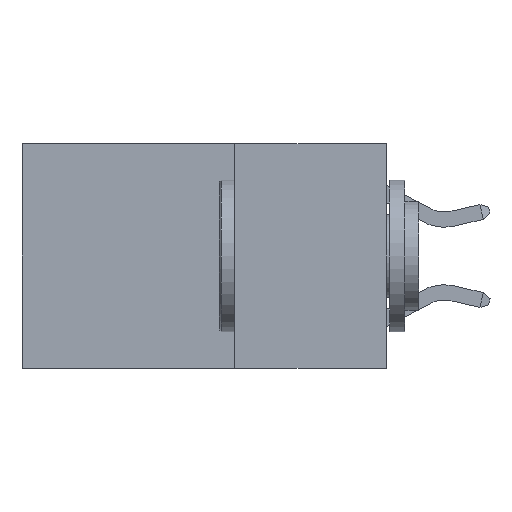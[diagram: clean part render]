
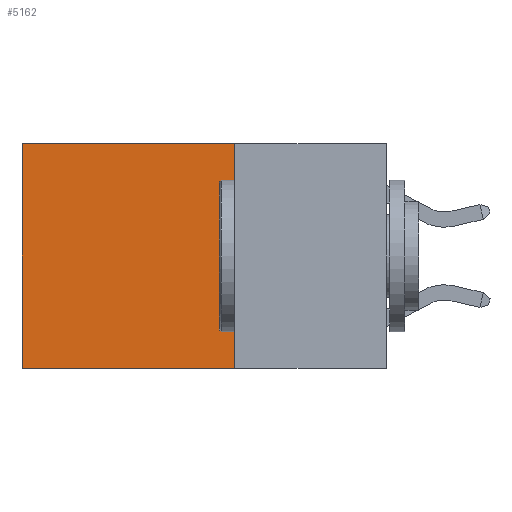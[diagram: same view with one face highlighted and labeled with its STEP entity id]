
A CAD part, left-side view. The second image highlights one B-rep face of the part: STEP entity #5162.
In plain terms, the highlighted planar face has unit normal (-1, 0, 0).
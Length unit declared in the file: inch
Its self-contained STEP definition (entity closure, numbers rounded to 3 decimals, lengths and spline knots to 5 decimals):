
#210 = EDGE_CURVE ( 'NONE', #7461, #4934, #9469, .T. ) ;
#253 = CARTESIAN_POINT ( 'NONE',  ( 0.2625, 0.25, -0.37 ) ) ;
#627 = CARTESIAN_POINT ( 'NONE',  ( 0.2625, 0.6, 0. ) ) ;
#638 = CARTESIAN_POINT ( 'NONE',  ( 0.2625, 0.6, 0. ) ) ;
#1052 = ORIENTED_EDGE ( 'NONE', *, *, #5320, .F. ) ;
#1684 = DIRECTION ( 'NONE',  ( 0., 0., -1. ) ) ;
#1700 = PLANE ( 'NONE',  #1705 ) ;
#1705 = AXIS2_PLACEMENT_3D ( 'NONE', #1714, #1871, #1684 ) ;
#1714 = CARTESIAN_POINT ( 'NONE',  ( 0.2625, 0.25, 0. ) ) ;
#1727 = VERTEX_POINT ( 'NONE', #5389 ) ;
#1871 = DIRECTION ( 'NONE',  ( 1., 0., 0. ) ) ;
#3187 = ORIENTED_EDGE ( 'NONE', *, *, #8732, .F. ) ;
#3204 = LINE ( 'NONE', #253, #3427 ) ;
#3427 = VECTOR ( 'NONE', #5504, 39.37008 ) ;
#3429 = VECTOR ( 'NONE', #3746, 39.37008 ) ;
#3746 = DIRECTION ( 'NONE',  ( 0., 1., 0. ) ) ;
#3990 = ORIENTED_EDGE ( 'NONE', *, *, #210, .T. ) ;
#4029 = CARTESIAN_POINT ( 'NONE',  ( 0.2625, 0.25, 0. ) ) ;
#4235 = DIRECTION ( 'NONE',  ( 0., 0., -1. ) ) ;
#4585 = CARTESIAN_POINT ( 'NONE',  ( 0.2625, 0.25, 0. ) ) ;
#4934 = VERTEX_POINT ( 'NONE', #8259 ) ;
#5162 = ADVANCED_FACE ( 'NONE', ( #8408 ), #1700, .F. ) ;
#5320 = EDGE_CURVE ( 'NONE', #1727, #4934, #3204, .T. ) ;
#5389 = CARTESIAN_POINT ( 'NONE',  ( 0.2625, 0.25, -0.37 ) ) ;
#5504 = DIRECTION ( 'NONE',  ( 0., 1., 0. ) ) ;
#7113 = VECTOR ( 'NONE', #7655, 39.37008 ) ;
#7322 = LINE ( 'NONE', #9468, #3429 ) ;
#7461 = VERTEX_POINT ( 'NONE', #638 ) ;
#7625 = VECTOR ( 'NONE', #4235, 39.37008 ) ;
#7630 = VERTEX_POINT ( 'NONE', #4585 ) ;
#7655 = DIRECTION ( 'NONE',  ( 0., 0., -1. ) ) ;
#8087 = EDGE_LOOP ( 'NONE', ( #3990, #1052, #3187, #8374 ) ) ;
#8259 = CARTESIAN_POINT ( 'NONE',  ( 0.2625, 0.6, -0.37 ) ) ;
#8374 = ORIENTED_EDGE ( 'NONE', *, *, #9227, .T. ) ;
#8408 = FACE_OUTER_BOUND ( 'NONE', #8087, .T. ) ;
#8732 = EDGE_CURVE ( 'NONE', #7630, #1727, #8982, .T. ) ;
#8982 = LINE ( 'NONE', #4029, #7113 ) ;
#9227 = EDGE_CURVE ( 'NONE', #7630, #7461, #7322, .T. ) ;
#9468 = CARTESIAN_POINT ( 'NONE',  ( 0.2625, 0.25, 0. ) ) ;
#9469 = LINE ( 'NONE', #627, #7625 ) ;
